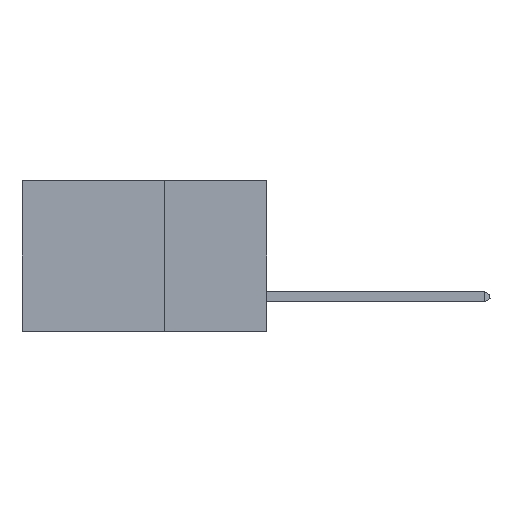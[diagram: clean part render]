
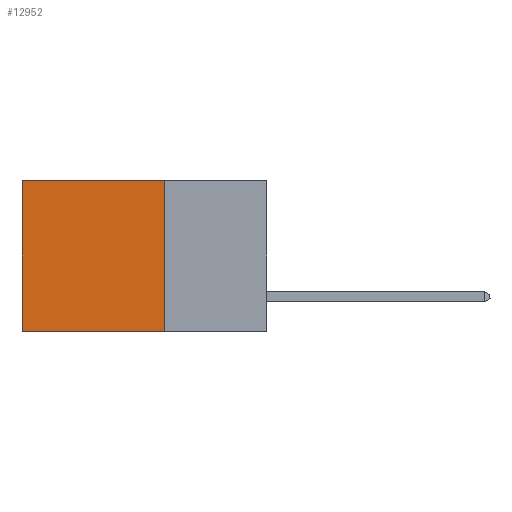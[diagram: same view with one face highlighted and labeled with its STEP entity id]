
A CAD part, left-side view. The second image highlights one B-rep face of the part: STEP entity #12952.
In plain terms, the highlighted planar face has unit normal (-1, 0, 0).
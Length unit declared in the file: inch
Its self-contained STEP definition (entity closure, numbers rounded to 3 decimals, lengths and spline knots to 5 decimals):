
#558 = VERTEX_POINT ( 'NONE', #17121 ) ;
#765 = PLANE ( 'NONE',  #15136 ) ;
#1173 = DIRECTION ( 'NONE',  ( 0., 0., -1. ) ) ;
#1510 = CARTESIAN_POINT ( 'NONE',  ( 0.2875, 0.25, 0. ) ) ;
#1884 = ORIENTED_EDGE ( 'NONE', *, *, #5321, .F. ) ;
#2276 = DIRECTION ( 'NONE',  ( 0., 1., 0. ) ) ;
#2699 = CARTESIAN_POINT ( 'NONE',  ( 0.2875, 0.25, 0. ) ) ;
#3175 = VERTEX_POINT ( 'NONE', #3306 ) ;
#3306 = CARTESIAN_POINT ( 'NONE',  ( 0.2875, 0.6, -0.37 ) ) ;
#3456 = CARTESIAN_POINT ( 'NONE',  ( 0.2875, 0.25, -0.37 ) ) ;
#3608 = CARTESIAN_POINT ( 'NONE',  ( 0.2875, 0.25, -0.37 ) ) ;
#3706 = VECTOR ( 'NONE', #2276, 39.37008 ) ;
#4037 = VECTOR ( 'NONE', #12283, 39.37008 ) ;
#4064 = VECTOR ( 'NONE', #1173, 39.37008 ) ;
#4513 = ORIENTED_EDGE ( 'NONE', *, *, #16782, .F. ) ;
#4729 = VECTOR ( 'NONE', #6412, 39.37008 ) ;
#5098 = CARTESIAN_POINT ( 'NONE',  ( 0.2875, 0.25, 0. ) ) ;
#5321 = EDGE_CURVE ( 'NONE', #15176, #17333, #10551, .T. ) ;
#5969 = DIRECTION ( 'NONE',  ( 1., 0., 0. ) ) ;
#6412 = DIRECTION ( 'NONE',  ( 0., 1., 0. ) ) ;
#7662 = CARTESIAN_POINT ( 'NONE',  ( 0.2875, 0.6, 0. ) ) ;
#9628 = FACE_OUTER_BOUND ( 'NONE', #11908, .T. ) ;
#10551 = LINE ( 'NONE', #2699, #4064 ) ;
#11467 = DIRECTION ( 'NONE',  ( 0., 0., -1. ) ) ;
#11908 = EDGE_LOOP ( 'NONE', ( #18039, #4513, #1884, #17420 ) ) ;
#12203 = EDGE_CURVE ( 'NONE', #558, #3175, #12301, .T. ) ;
#12283 = DIRECTION ( 'NONE',  ( 0., 0., -1. ) ) ;
#12301 = LINE ( 'NONE', #7662, #4037 ) ;
#12952 = ADVANCED_FACE ( 'NONE', ( #9628 ), #765, .F. ) ;
#14663 = EDGE_CURVE ( 'NONE', #15176, #558, #18526, .T. ) ;
#15136 = AXIS2_PLACEMENT_3D ( 'NONE', #1510, #5969, #11467 ) ;
#15176 = VERTEX_POINT ( 'NONE', #5098 ) ;
#15358 = CARTESIAN_POINT ( 'NONE',  ( 0.2875, 0.25, 0. ) ) ;
#16782 = EDGE_CURVE ( 'NONE', #17333, #3175, #17741, .T. ) ;
#17121 = CARTESIAN_POINT ( 'NONE',  ( 0.2875, 0.6, 0. ) ) ;
#17333 = VERTEX_POINT ( 'NONE', #3456 ) ;
#17420 = ORIENTED_EDGE ( 'NONE', *, *, #14663, .T. ) ;
#17741 = LINE ( 'NONE', #3608, #4729 ) ;
#18039 = ORIENTED_EDGE ( 'NONE', *, *, #12203, .T. ) ;
#18526 = LINE ( 'NONE', #15358, #3706 ) ;
